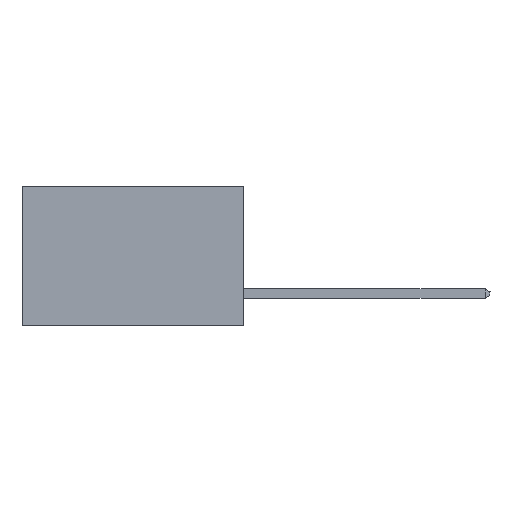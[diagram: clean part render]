
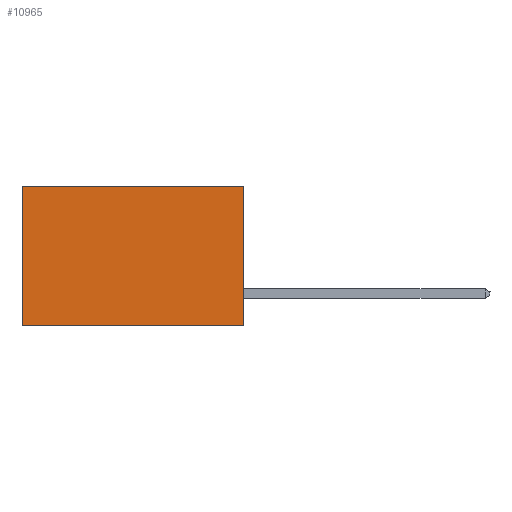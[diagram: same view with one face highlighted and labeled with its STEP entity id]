
A CAD part, left-side view. The second image highlights one B-rep face of the part: STEP entity #10965.
In plain terms, the highlighted planar face has unit normal (-1, 0, 0).
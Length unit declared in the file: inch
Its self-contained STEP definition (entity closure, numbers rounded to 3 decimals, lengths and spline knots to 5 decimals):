
#50 = ORIENTED_EDGE ( 'NONE', *, *, #12733, .F. ) ;
#1221 = DIRECTION ( 'NONE',  ( 1., 0., 0. ) ) ;
#1688 = CARTESIAN_POINT ( 'NONE',  ( 0.277, 0., 0. ) ) ;
#1735 = DIRECTION ( 'NONE',  ( 0., 1., 0. ) ) ;
#2108 = LINE ( 'NONE', #5765, #7893 ) ;
#2446 = CARTESIAN_POINT ( 'NONE',  ( 0.277, 0.59, -0.37 ) ) ;
#3029 = VECTOR ( 'NONE', #6515, 39.37008 ) ;
#3394 = LINE ( 'NONE', #5356, #3029 ) ;
#3958 = CARTESIAN_POINT ( 'NONE',  ( 0.277, 0., -0.37 ) ) ;
#4890 = ORIENTED_EDGE ( 'NONE', *, *, #12913, .F. ) ;
#5203 = VERTEX_POINT ( 'NONE', #12449 ) ;
#5356 = CARTESIAN_POINT ( 'NONE',  ( 0.277, 0., -0.37 ) ) ;
#5765 = CARTESIAN_POINT ( 'NONE',  ( 0.277, 0.59, -0.37 ) ) ;
#5888 = VECTOR ( 'NONE', #12014, 39.37008 ) ;
#6515 = DIRECTION ( 'NONE',  ( 0., 1., 0. ) ) ;
#7493 = EDGE_CURVE ( 'NONE', #8461, #14152, #2108, .T. ) ;
#7608 = VECTOR ( 'NONE', #1735, 39.37008 ) ;
#7785 = ORIENTED_EDGE ( 'NONE', *, *, #7493, .T. ) ;
#7893 = VECTOR ( 'NONE', #8020, 39.37008 ) ;
#7911 = ORIENTED_EDGE ( 'NONE', *, *, #13427, .T. ) ;
#8020 = DIRECTION ( 'NONE',  ( 0., 0., -1. ) ) ;
#8461 = VERTEX_POINT ( 'NONE', #13220 ) ;
#8885 = EDGE_LOOP ( 'NONE', ( #7785, #4890, #50, #7911 ) ) ;
#9013 = LINE ( 'NONE', #3958, #5888 ) ;
#9265 = DIRECTION ( 'NONE',  ( 0., 0., -1. ) ) ;
#9273 = FACE_OUTER_BOUND ( 'NONE', #8885, .T. ) ;
#9838 = AXIS2_PLACEMENT_3D ( 'NONE', #11542, #1221, #9265 ) ;
#10373 = PLANE ( 'NONE',  #9838 ) ;
#10916 = CARTESIAN_POINT ( 'NONE',  ( 0.277, 0., -0.37 ) ) ;
#10965 = ADVANCED_FACE ( 'NONE', ( #9273 ), #10373, .F. ) ;
#11542 = CARTESIAN_POINT ( 'NONE',  ( 0.277, 0., -0.37 ) ) ;
#12014 = DIRECTION ( 'NONE',  ( 0., 0., -1. ) ) ;
#12449 = CARTESIAN_POINT ( 'NONE',  ( 0.277, 0., 0. ) ) ;
#12526 = VERTEX_POINT ( 'NONE', #10916 ) ;
#12733 = EDGE_CURVE ( 'NONE', #5203, #12526, #9013, .T. ) ;
#12913 = EDGE_CURVE ( 'NONE', #12526, #14152, #3394, .T. ) ;
#13220 = CARTESIAN_POINT ( 'NONE',  ( 0.277, 0.59, 0. ) ) ;
#13427 = EDGE_CURVE ( 'NONE', #5203, #8461, #13635, .T. ) ;
#13635 = LINE ( 'NONE', #1688, #7608 ) ;
#14152 = VERTEX_POINT ( 'NONE', #2446 ) ;
